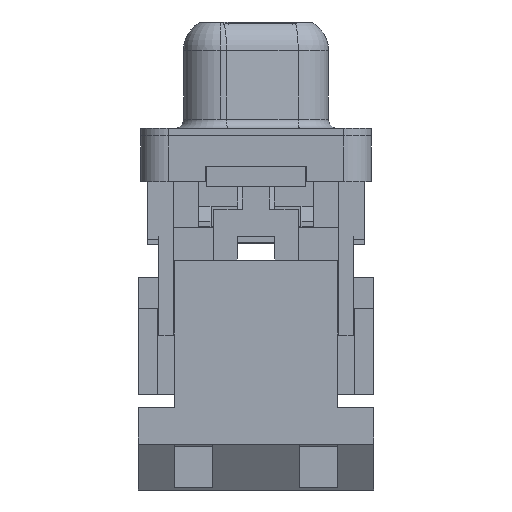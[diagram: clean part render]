
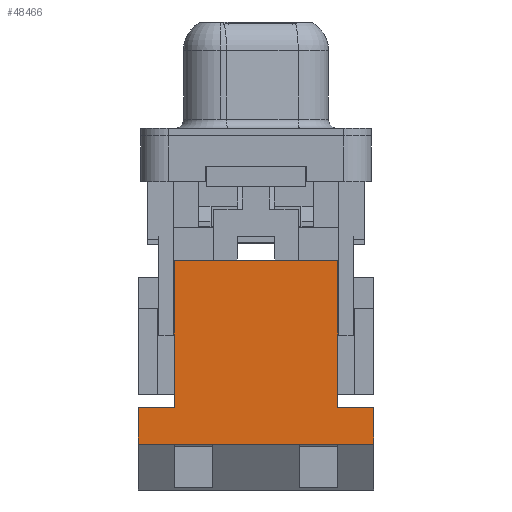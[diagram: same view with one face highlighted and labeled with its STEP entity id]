
A CAD part, left-side view. The second image highlights one B-rep face of the part: STEP entity #48466.
In plain terms, the highlighted planar face has unit normal (-1, 0, 0).
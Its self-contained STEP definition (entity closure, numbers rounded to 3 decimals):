
#1020 = VERTEX_POINT ( 'NONE', #36847 ) ;
#1414 = DIRECTION ( 'NONE',  ( 0., 0., -1. ) ) ;
#1625 = DIRECTION ( 'NONE',  ( 0., 0., -1. ) ) ;
#1662 = DIRECTION ( 'NONE',  ( 1., 0., 0. ) ) ;
#1926 = PLANE ( 'NONE',  #47307 ) ;
#2086 = EDGE_LOOP ( 'NONE', ( #32557, #54761, #22339, #13999, #53241, #29925, #2725, #40999 ) ) ;
#2219 = VERTEX_POINT ( 'NONE', #47808 ) ;
#2247 = VECTOR ( 'NONE', #6698, 1000. ) ;
#2725 = ORIENTED_EDGE ( 'NONE', *, *, #22259, .T. ) ;
#6645 = DIRECTION ( 'NONE',  ( 0., 0., -1. ) ) ;
#6698 = DIRECTION ( 'NONE',  ( 0., -1., 0. ) ) ;
#7891 = EDGE_CURVE ( 'NONE', #12439, #2219, #22014, .T. ) ;
#8570 = CARTESIAN_POINT ( 'NONE',  ( 3.245, -6.425, -16.8 ) ) ;
#9217 = CARTESIAN_POINT ( 'NONE',  ( 3.245, 6.425, -15.3 ) ) ;
#9678 = DIRECTION ( 'NONE',  ( 0., -1., 0. ) ) ;
#10507 = EDGE_CURVE ( 'NONE', #42558, #15096, #40304, .T. ) ;
#11333 = VERTEX_POINT ( 'NONE', #36757 ) ;
#12439 = VERTEX_POINT ( 'NONE', #8570 ) ;
#13582 = LINE ( 'NONE', #47232, #51665 ) ;
#13700 = EDGE_CURVE ( 'NONE', #32353, #42558, #13582, .T. ) ;
#13960 = VECTOR ( 'NONE', #1414, 1000. ) ;
#13999 = ORIENTED_EDGE ( 'NONE', *, *, #44723, .F. ) ;
#14151 = LINE ( 'NONE', #27490, #45997 ) ;
#14966 = LINE ( 'NONE', #9217, #13960 ) ;
#15096 = VERTEX_POINT ( 'NONE', #27480 ) ;
#17204 = CARTESIAN_POINT ( 'NONE',  ( 3.245, -4.45, -6.8 ) ) ;
#19156 = CARTESIAN_POINT ( 'NONE',  ( 3.245, -6.425, -15.3 ) ) ;
#19545 = LINE ( 'NONE', #54046, #36834 ) ;
#22014 = LINE ( 'NONE', #34523, #43741 ) ;
#22259 = EDGE_CURVE ( 'NONE', #32353, #11333, #14151, .T. ) ;
#22339 = ORIENTED_EDGE ( 'NONE', *, *, #47306, .F. ) ;
#22816 = FACE_OUTER_BOUND ( 'NONE', #2086, .T. ) ;
#23082 = CARTESIAN_POINT ( 'NONE',  ( 3.245, -4.45, -6.8 ) ) ;
#27480 = CARTESIAN_POINT ( 'NONE',  ( 3.245, -4.45, -14.8 ) ) ;
#27490 = CARTESIAN_POINT ( 'NONE',  ( 3.245, 4.45, -6.8 ) ) ;
#29925 = ORIENTED_EDGE ( 'NONE', *, *, #13700, .F. ) ;
#30512 = CARTESIAN_POINT ( 'NONE',  ( 3.245, 4.45, -6.8 ) ) ;
#31689 = LINE ( 'NONE', #19156, #51765 ) ;
#32353 = VERTEX_POINT ( 'NONE', #30512 ) ;
#32557 = ORIENTED_EDGE ( 'NONE', *, *, #54488, .T. ) ;
#33978 = DIRECTION ( 'NONE',  ( 0., 1., 0. ) ) ;
#34523 = CARTESIAN_POINT ( 'NONE',  ( 3.245, -6.425, -16.8 ) ) ;
#35027 = DIRECTION ( 'NONE',  ( 0., 0., -1. ) ) ;
#36185 = CARTESIAN_POINT ( 'NONE',  ( 3.245, 6.425, -14.8 ) ) ;
#36757 = CARTESIAN_POINT ( 'NONE',  ( 3.245, 4.45, -14.8 ) ) ;
#36834 = VECTOR ( 'NONE', #53494, 1000. ) ;
#36847 = CARTESIAN_POINT ( 'NONE',  ( 3.245, -6.425, -14.8 ) ) ;
#38318 = CARTESIAN_POINT ( 'NONE',  ( 3.245, 6.425, -14.8 ) ) ;
#39767 = CARTESIAN_POINT ( 'NONE',  ( 3.245, -6.425, -15.3 ) ) ;
#40304 = LINE ( 'NONE', #23082, #52871 ) ;
#40579 = DIRECTION ( 'NONE',  ( 0., 0., -1. ) ) ;
#40999 = ORIENTED_EDGE ( 'NONE', *, *, #45106, .F. ) ;
#42558 = VERTEX_POINT ( 'NONE', #17204 ) ;
#43741 = VECTOR ( 'NONE', #33978, 1000. ) ;
#44723 = EDGE_CURVE ( 'NONE', #15096, #1020, #19545, .T. ) ;
#45106 = EDGE_CURVE ( 'NONE', #47540, #11333, #53703, .T. ) ;
#45997 = VECTOR ( 'NONE', #1625, 1000. ) ;
#47232 = CARTESIAN_POINT ( 'NONE',  ( 3.245, 4.45, -6.8 ) ) ;
#47306 = EDGE_CURVE ( 'NONE', #1020, #12439, #31689, .T. ) ;
#47307 = AXIS2_PLACEMENT_3D ( 'NONE', #39767, #1662, #40579 ) ;
#47540 = VERTEX_POINT ( 'NONE', #38318 ) ;
#47808 = CARTESIAN_POINT ( 'NONE',  ( 3.245, 6.425, -16.8 ) ) ;
#48466 = ADVANCED_FACE ( 'NONE', ( #22816 ), #1926, .F. ) ;
#51665 = VECTOR ( 'NONE', #9678, 1000. ) ;
#51765 = VECTOR ( 'NONE', #35027, 1000. ) ;
#52871 = VECTOR ( 'NONE', #6645, 1000. ) ;
#53241 = ORIENTED_EDGE ( 'NONE', *, *, #10507, .F. ) ;
#53494 = DIRECTION ( 'NONE',  ( 0., -1., 0. ) ) ;
#53703 = LINE ( 'NONE', #36185, #2247 ) ;
#54046 = CARTESIAN_POINT ( 'NONE',  ( 3.245, 6.425, -14.8 ) ) ;
#54488 = EDGE_CURVE ( 'NONE', #47540, #2219, #14966, .T. ) ;
#54761 = ORIENTED_EDGE ( 'NONE', *, *, #7891, .F. ) ;
